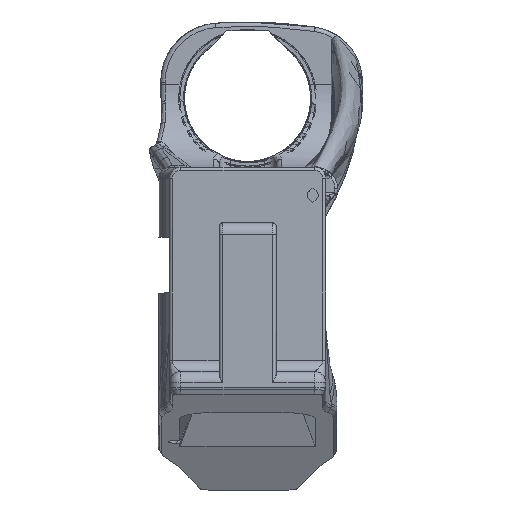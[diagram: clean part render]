
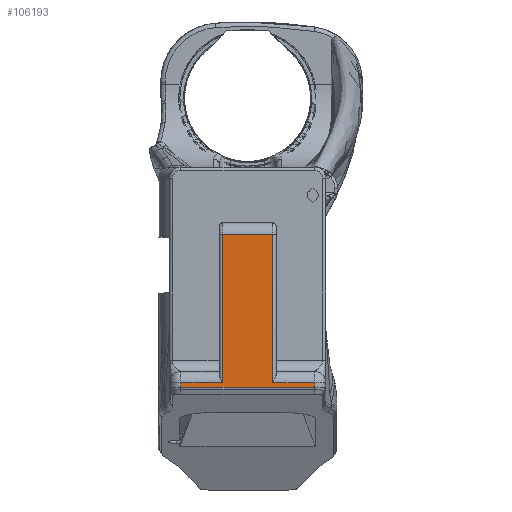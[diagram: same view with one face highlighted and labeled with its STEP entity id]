
A CAD part, top view. The second image highlights one B-rep face of the part: STEP entity #106193.
In plain terms, the highlighted planar face has unit normal (0, 0, 1).
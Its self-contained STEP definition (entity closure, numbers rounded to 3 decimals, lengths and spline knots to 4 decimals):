
#2774 = CARTESIAN_POINT ( 'NONE',  ( 0.255, -0.6, 6.65 ) ) ;
#5813 = DIRECTION ( 'NONE',  ( 0., 1., 0. ) ) ;
#19676 = VECTOR ( 'NONE', #240234, 39.3701 ) ;
#23869 = EDGE_CURVE ( 'NONE', #41303, #32726, #110248, .T. ) ;
#26517 = DIRECTION ( 'NONE',  ( 0., -1., 0. ) ) ;
#29079 = VECTOR ( 'NONE', #26517, 39.3701 ) ;
#32207 = CARTESIAN_POINT ( 'NONE',  ( 0.255, -1.9323, 6.65 ) ) ;
#32726 = VERTEX_POINT ( 'NONE', #238932 ) ;
#32752 = EDGE_CURVE ( 'NONE', #115160, #94842, #64028, .T. ) ;
#33267 = CARTESIAN_POINT ( 'NONE',  ( 0.6, -1.9765, 6.65 ) ) ;
#41303 = VERTEX_POINT ( 'NONE', #115805 ) ;
#46629 = LINE ( 'NONE', #122844, #19676 ) ;
#48793 = EDGE_LOOP ( 'NONE', ( #233384, #105926, #228970, #66140, #164639, #78477, #83944, #53947 ) ) ;
#53947 = ORIENTED_EDGE ( 'NONE', *, *, #229667, .T. ) ;
#55239 = EDGE_CURVE ( 'NONE', #94842, #169943, #66673, .T. ) ;
#58205 = DIRECTION ( 'NONE',  ( 0., 1., 0. ) ) ;
#64028 = LINE ( 'NONE', #121492, #29079 ) ;
#66140 = ORIENTED_EDGE ( 'NONE', *, *, #221281, .T. ) ;
#66673 = LINE ( 'NONE', #142899, #86129 ) ;
#78342 = PLANE ( 'NONE',  #108924 ) ;
#78477 = ORIENTED_EDGE ( 'NONE', *, *, #219115, .T. ) ;
#79100 = VECTOR ( 'NONE', #244531, 39.3701 ) ;
#83944 = ORIENTED_EDGE ( 'NONE', *, *, #86672, .T. ) ;
#86129 = VECTOR ( 'NONE', #219129, 39.3701 ) ;
#86672 = EDGE_CURVE ( 'NONE', #159012, #182327, #157426, .T. ) ;
#94842 = VERTEX_POINT ( 'NONE', #213874 ) ;
#98163 = LINE ( 'NONE', #211872, #227112 ) ;
#105926 = ORIENTED_EDGE ( 'NONE', *, *, #55239, .T. ) ;
#106193 = ADVANCED_FACE ( 'NONE', ( #118313 ), #78342, .F. ) ;
#108924 = AXIS2_PLACEMENT_3D ( 'NONE', #229546, #195750, #5813 ) ;
#110248 = LINE ( 'NONE', #165264, #111839 ) ;
#111839 = VECTOR ( 'NONE', #201545, 39.3701 ) ;
#115160 = VERTEX_POINT ( 'NONE', #161750 ) ;
#115805 = CARTESIAN_POINT ( 'NONE',  ( 0.225, -1.9323, 6.65 ) ) ;
#118313 = FACE_OUTER_BOUND ( 'NONE', #48793, .T. ) ;
#119057 = VECTOR ( 'NONE', #193933, 39.3701 ) ;
#121492 = CARTESIAN_POINT ( 'NONE',  ( -0.6, -2.0323, 6.65 ) ) ;
#122844 = CARTESIAN_POINT ( 'NONE',  ( 0.255, -1.9323, 6.65 ) ) ;
#125899 = CARTESIAN_POINT ( 'NONE',  ( -0.225, -0.6, 6.65 ) ) ;
#139911 = DIRECTION ( 'NONE',  ( 0., -1., 0. ) ) ;
#142899 = CARTESIAN_POINT ( 'NONE',  ( 0.6, -1.9765, 6.65 ) ) ;
#157426 = LINE ( 'NONE', #233644, #225468 ) ;
#159012 = VERTEX_POINT ( 'NONE', #125899 ) ;
#161750 = CARTESIAN_POINT ( 'NONE',  ( -0.6, -1.9323, 6.65 ) ) ;
#164639 = ORIENTED_EDGE ( 'NONE', *, *, #23869, .T. ) ;
#165264 = CARTESIAN_POINT ( 'NONE',  ( 0.225, -2.0323, 6.65 ) ) ;
#165879 = LINE ( 'NONE', #32207, #79100 ) ;
#167379 = VERTEX_POINT ( 'NONE', #226782 ) ;
#169943 = VERTEX_POINT ( 'NONE', #33267 ) ;
#173946 = LINE ( 'NONE', #2774, #119057 ) ;
#182327 = VERTEX_POINT ( 'NONE', #192849 ) ;
#192849 = CARTESIAN_POINT ( 'NONE',  ( -0.225, -1.9323, 6.65 ) ) ;
#193933 = DIRECTION ( 'NONE',  ( -1., 0., 0. ) ) ;
#195750 = DIRECTION ( 'NONE',  ( 0., 0., -1. ) ) ;
#201545 = DIRECTION ( 'NONE',  ( 0., 1., 0. ) ) ;
#211872 = CARTESIAN_POINT ( 'NONE',  ( 0.6, -1.8323, 6.65 ) ) ;
#213874 = CARTESIAN_POINT ( 'NONE',  ( -0.6, -1.9765, 6.65 ) ) ;
#219115 = EDGE_CURVE ( 'NONE', #32726, #159012, #173946, .T. ) ;
#219129 = DIRECTION ( 'NONE',  ( 1., 0., 0. ) ) ;
#221281 = EDGE_CURVE ( 'NONE', #167379, #41303, #165879, .T. ) ;
#225468 = VECTOR ( 'NONE', #139911, 39.3701 ) ;
#226782 = CARTESIAN_POINT ( 'NONE',  ( 0.6, -1.9323, 6.65 ) ) ;
#227112 = VECTOR ( 'NONE', #58205, 39.3701 ) ;
#228745 = EDGE_CURVE ( 'NONE', #169943, #167379, #98163, .T. ) ;
#228970 = ORIENTED_EDGE ( 'NONE', *, *, #228745, .T. ) ;
#229546 = CARTESIAN_POINT ( 'NONE',  ( 0.255, -2.0323, 6.65 ) ) ;
#229667 = EDGE_CURVE ( 'NONE', #182327, #115160, #46629, .T. ) ;
#233384 = ORIENTED_EDGE ( 'NONE', *, *, #32752, .T. ) ;
#233644 = CARTESIAN_POINT ( 'NONE',  ( -0.225, -1.8323, 6.65 ) ) ;
#238932 = CARTESIAN_POINT ( 'NONE',  ( 0.225, -0.6, 6.65 ) ) ;
#240234 = DIRECTION ( 'NONE',  ( -1., 0., 0. ) ) ;
#244531 = DIRECTION ( 'NONE',  ( -1., 0., 0. ) ) ;
